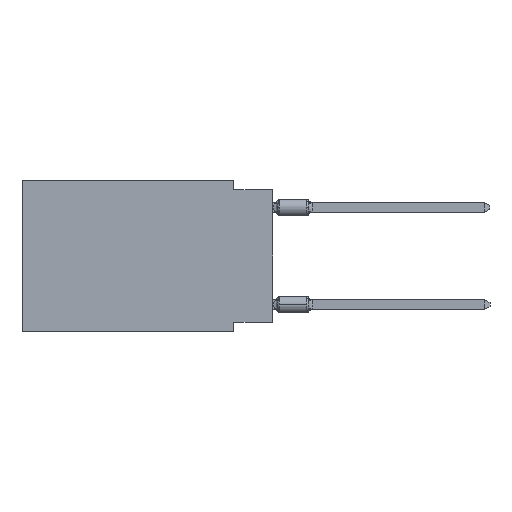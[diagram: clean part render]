
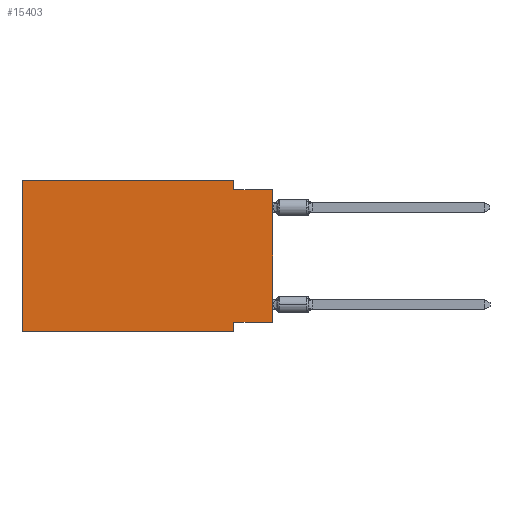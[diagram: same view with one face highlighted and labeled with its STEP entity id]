
A CAD part, left-side view. The second image highlights one B-rep face of the part: STEP entity #15403.
In plain terms, the highlighted planar face has unit normal (-1, 0, 0).
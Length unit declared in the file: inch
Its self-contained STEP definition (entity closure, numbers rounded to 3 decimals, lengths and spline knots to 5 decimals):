
#223 = CARTESIAN_POINT ( 'NONE',  ( 0., 0.1, -0.365 ) ) ;
#842 = CARTESIAN_POINT ( 'NONE',  ( 0., 0., -0.025 ) ) ;
#940 = LINE ( 'NONE', #17573, #6207 ) ;
#1309 = DIRECTION ( 'NONE',  ( 0., -1., 0. ) ) ;
#1641 = EDGE_CURVE ( 'NONE', #10606, #11128, #3943, .T. ) ;
#2073 = CARTESIAN_POINT ( 'NONE',  ( 0., 0., -0.365 ) ) ;
#2091 = ORIENTED_EDGE ( 'NONE', *, *, #16350, .T. ) ;
#2216 = VECTOR ( 'NONE', #17062, 39.37008 ) ;
#2357 = DIRECTION ( 'NONE',  ( 0., 0., 1. ) ) ;
#2554 = VERTEX_POINT ( 'NONE', #7305 ) ;
#2923 = ORIENTED_EDGE ( 'NONE', *, *, #12455, .F. ) ;
#3943 = LINE ( 'NONE', #22561, #13906 ) ;
#4184 = CARTESIAN_POINT ( 'NONE',  ( 0., 0., 0. ) ) ;
#5061 = CARTESIAN_POINT ( 'NONE',  ( 0., 0.645, 0. ) ) ;
#5475 = ORIENTED_EDGE ( 'NONE', *, *, #1641, .F. ) ;
#5782 = CARTESIAN_POINT ( 'NONE',  ( 0., 0.645, -0.39 ) ) ;
#6207 = VECTOR ( 'NONE', #15516, 39.37008 ) ;
#6657 = CARTESIAN_POINT ( 'NONE',  ( 0., 0.1, -0.025 ) ) ;
#7029 = VERTEX_POINT ( 'NONE', #5061 ) ;
#7068 = DIRECTION ( 'NONE',  ( 0., 0., -1. ) ) ;
#7110 = EDGE_CURVE ( 'NONE', #14100, #14386, #11169, .T. ) ;
#7305 = CARTESIAN_POINT ( 'NONE',  ( 0., 0.1, 0. ) ) ;
#8780 = ORIENTED_EDGE ( 'NONE', *, *, #16096, .F. ) ;
#8919 = CARTESIAN_POINT ( 'NONE',  ( 0., 0.1, 0. ) ) ;
#8993 = VECTOR ( 'NONE', #21849, 39.37008 ) ;
#10606 = VERTEX_POINT ( 'NONE', #2073 ) ;
#10991 = ORIENTED_EDGE ( 'NONE', *, *, #18242, .F. ) ;
#11128 = VERTEX_POINT ( 'NONE', #223 ) ;
#11169 = LINE ( 'NONE', #5782, #2216 ) ;
#11249 = FACE_OUTER_BOUND ( 'NONE', #12752, .T. ) ;
#12455 = EDGE_CURVE ( 'NONE', #23790, #23275, #940, .T. ) ;
#12560 = CARTESIAN_POINT ( 'NONE',  ( 0., 0.645, 0. ) ) ;
#12752 = EDGE_LOOP ( 'NONE', ( #2091, #2923, #13588, #17277, #10991, #24073, #8780, #5475 ) ) ;
#13588 = ORIENTED_EDGE ( 'NONE', *, *, #16928, .F. ) ;
#13906 = VECTOR ( 'NONE', #14993, 39.37008 ) ;
#14079 = AXIS2_PLACEMENT_3D ( 'NONE', #14963, #22408, #17024 ) ;
#14100 = VERTEX_POINT ( 'NONE', #16142 ) ;
#14386 = VERTEX_POINT ( 'NONE', #21508 ) ;
#14532 = EDGE_CURVE ( 'NONE', #7029, #2554, #19906, .T. ) ;
#14915 = VECTOR ( 'NONE', #2357, 39.37008 ) ;
#14963 = CARTESIAN_POINT ( 'NONE',  ( 0., 0.645, 0. ) ) ;
#14993 = DIRECTION ( 'NONE',  ( 0., 1., 0. ) ) ;
#15403 = ADVANCED_FACE ( 'NONE', ( #11249 ), #18482, .F. ) ;
#15495 = CARTESIAN_POINT ( 'NONE',  ( 0., 0.645, 0. ) ) ;
#15516 = DIRECTION ( 'NONE',  ( 0., -1., 0. ) ) ;
#15722 = DIRECTION ( 'NONE',  ( 0., 0., 1. ) ) ;
#15819 = LINE ( 'NONE', #4184, #14915 ) ;
#16096 = EDGE_CURVE ( 'NONE', #11128, #14386, #16576, .T. ) ;
#16142 = CARTESIAN_POINT ( 'NONE',  ( 0., 0.645, -0.39 ) ) ;
#16350 = EDGE_CURVE ( 'NONE', #10606, #23275, #15819, .T. ) ;
#16576 = LINE ( 'NONE', #23802, #8993 ) ;
#16928 = EDGE_CURVE ( 'NONE', #2554, #23790, #19704, .T. ) ;
#17024 = DIRECTION ( 'NONE',  ( 0., 0., -1. ) ) ;
#17062 = DIRECTION ( 'NONE',  ( 0., -1., 0. ) ) ;
#17277 = ORIENTED_EDGE ( 'NONE', *, *, #14532, .F. ) ;
#17573 = CARTESIAN_POINT ( 'NONE',  ( 0., 0., -0.025 ) ) ;
#18242 = EDGE_CURVE ( 'NONE', #14100, #7029, #21349, .T. ) ;
#18327 = VECTOR ( 'NONE', #1309, 39.37008 ) ;
#18482 = PLANE ( 'NONE',  #14079 ) ;
#19635 = VECTOR ( 'NONE', #15722, 39.37008 ) ;
#19704 = LINE ( 'NONE', #8919, #22722 ) ;
#19906 = LINE ( 'NONE', #12560, #18327 ) ;
#21349 = LINE ( 'NONE', #15495, #19635 ) ;
#21508 = CARTESIAN_POINT ( 'NONE',  ( 0., 0.1, -0.39 ) ) ;
#21849 = DIRECTION ( 'NONE',  ( 0., 0., -1. ) ) ;
#22408 = DIRECTION ( 'NONE',  ( 1., 0., 0. ) ) ;
#22561 = CARTESIAN_POINT ( 'NONE',  ( 0., 0., -0.365 ) ) ;
#22722 = VECTOR ( 'NONE', #7068, 39.37008 ) ;
#23275 = VERTEX_POINT ( 'NONE', #842 ) ;
#23790 = VERTEX_POINT ( 'NONE', #6657 ) ;
#23802 = CARTESIAN_POINT ( 'NONE',  ( 0., 0.1, -0.39 ) ) ;
#24073 = ORIENTED_EDGE ( 'NONE', *, *, #7110, .T. ) ;
